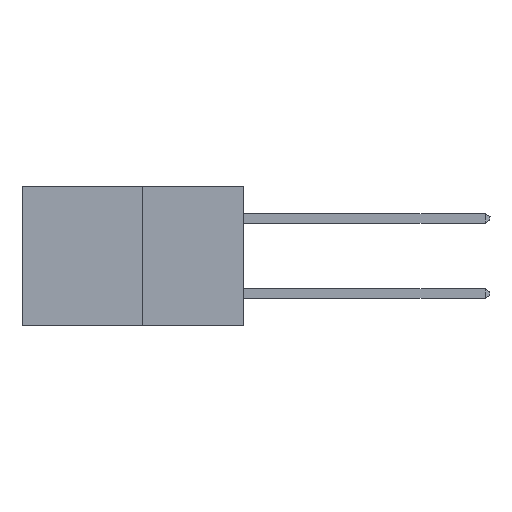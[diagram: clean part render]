
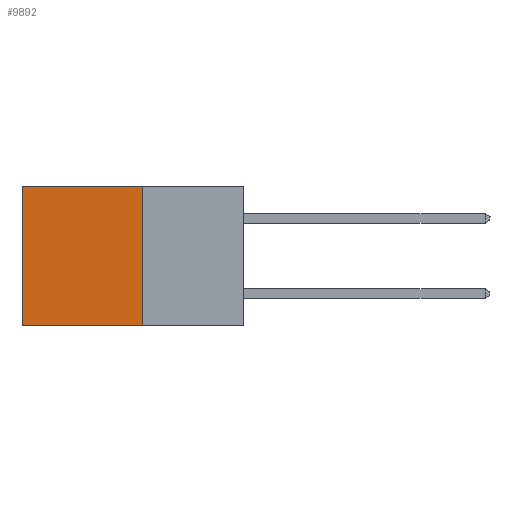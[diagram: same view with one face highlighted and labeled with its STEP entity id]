
A CAD part, left-side view. The second image highlights one B-rep face of the part: STEP entity #9892.
In plain terms, the highlighted planar face has unit normal (-1, 0, 0).
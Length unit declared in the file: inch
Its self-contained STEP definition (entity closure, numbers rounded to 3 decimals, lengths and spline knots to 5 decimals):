
#944 = LINE ( 'NONE', #29518, #15279 ) ;
#1964 = PLANE ( 'NONE',  #11809 ) ;
#2175 = EDGE_CURVE ( 'NONE', #6914, #32204, #27765, .T. ) ;
#2329 = CARTESIAN_POINT ( 'NONE',  ( 0.277, 0.59, -0.37 ) ) ;
#4102 = ORIENTED_EDGE ( 'NONE', *, *, #20802, .T. ) ;
#4667 = DIRECTION ( 'NONE',  ( 1., 0., 0. ) ) ;
#5250 = CARTESIAN_POINT ( 'NONE',  ( 0.277, 0.27, -0.37 ) ) ;
#5888 = VERTEX_POINT ( 'NONE', #14998 ) ;
#6914 = VERTEX_POINT ( 'NONE', #16097 ) ;
#7292 = ORIENTED_EDGE ( 'NONE', *, *, #2175, .T. ) ;
#9892 = ADVANCED_FACE ( 'NONE', ( #14313 ), #1964, .F. ) ;
#11016 = DIRECTION ( 'NONE',  ( 0., 1., 0. ) ) ;
#11320 = EDGE_LOOP ( 'NONE', ( #7292, #16683, #13306, #4102 ) ) ;
#11809 = AXIS2_PLACEMENT_3D ( 'NONE', #20745, #4667, #23405 ) ;
#13306 = ORIENTED_EDGE ( 'NONE', *, *, #20104, .F. ) ;
#13725 = VECTOR ( 'NONE', #21487, 39.37008 ) ;
#14313 = FACE_OUTER_BOUND ( 'NONE', #11320, .T. ) ;
#14998 = CARTESIAN_POINT ( 'NONE',  ( 0.277, 0.27, 0. ) ) ;
#15279 = VECTOR ( 'NONE', #11016, 39.37008 ) ;
#15713 = CARTESIAN_POINT ( 'NONE',  ( 0.277, 0.27, -0.37 ) ) ;
#16097 = CARTESIAN_POINT ( 'NONE',  ( 0.277, 0.59, 0. ) ) ;
#16683 = ORIENTED_EDGE ( 'NONE', *, *, #25787, .F. ) ;
#16901 = VECTOR ( 'NONE', #33995, 39.37008 ) ;
#18852 = DIRECTION ( 'NONE',  ( 0., 1., 0. ) ) ;
#20104 = EDGE_CURVE ( 'NONE', #5888, #22151, #30808, .T. ) ;
#20745 = CARTESIAN_POINT ( 'NONE',  ( 0.277, 0.27, -0.37 ) ) ;
#20802 = EDGE_CURVE ( 'NONE', #5888, #6914, #28707, .T. ) ;
#21487 = DIRECTION ( 'NONE',  ( 0., 0., -1. ) ) ;
#21794 = VECTOR ( 'NONE', #18852, 39.37008 ) ;
#22151 = VERTEX_POINT ( 'NONE', #5250 ) ;
#23405 = DIRECTION ( 'NONE',  ( 0., 0., -1. ) ) ;
#25787 = EDGE_CURVE ( 'NONE', #22151, #32204, #944, .T. ) ;
#26623 = CARTESIAN_POINT ( 'NONE',  ( 0.277, 0.59, -0.37 ) ) ;
#27765 = LINE ( 'NONE', #26623, #13725 ) ;
#28707 = LINE ( 'NONE', #31851, #21794 ) ;
#29518 = CARTESIAN_POINT ( 'NONE',  ( 0.277, 0.27, -0.37 ) ) ;
#30808 = LINE ( 'NONE', #15713, #16901 ) ;
#31851 = CARTESIAN_POINT ( 'NONE',  ( 0.277, 0.27, 0. ) ) ;
#32204 = VERTEX_POINT ( 'NONE', #2329 ) ;
#33995 = DIRECTION ( 'NONE',  ( 0., 0., -1. ) ) ;
